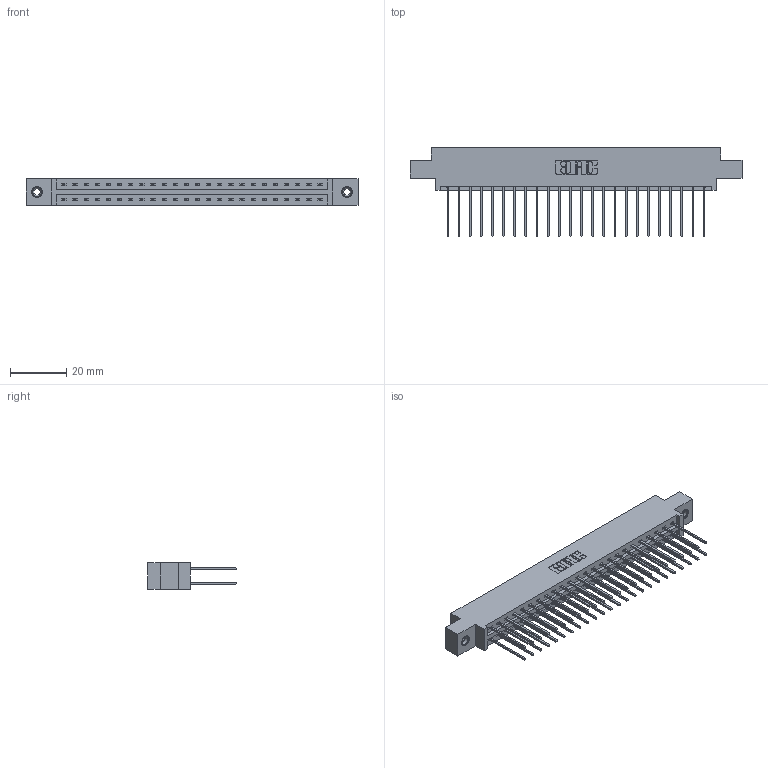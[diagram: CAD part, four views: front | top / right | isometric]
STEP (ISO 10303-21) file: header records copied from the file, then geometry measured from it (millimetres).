
FILE_DESCRIPTION (( 'STEP AP203' ), '1' );
FILE_NAME ('387-048-542-808.STEP', '2019-10-18T10:04:23', ( '' ), ( '' ), 'SwSTEP 2.0', 'SolidWorks 2016', '' );
FILE_SCHEMA (( 'CONFIG_CONTROL_DESIGN' ));
Length unit declared in the file: inch
Products named in the file (4): 345-292-001_345-293-142; 387-048-542-808; 337 Part_0.170 Offset - 0.156 Dia-TI; 345-250-001_345-250-003-102
Assembly tree (51 placements, depth 2):
  387-048-542-808
    337 Part_0.170 Offset - 0.156 Dia-TI
    345-292-001_345-293-142  x48
    345-250-001_345-250-003-102  x2
Bounding box: 118.11 x 31.63 x 9.4 mm (x, y, z)
Volume: 12307.5 mm3; surface area: 14986.1 mm2
Topology: 51 solids, 51 shells, 2770 faces, 8187 edges, 5386 vertices
Faces by surface type: plane 1930, cylinder 824, cone 12, torus 4
Entity records: 22272 total; most frequent: CARTESIAN_POINT 3749, ORIENTED_EDGE 3678, DIRECTION 3253, EDGE_CURVE 1839, VECTOR 1691, LINE 1691, VERTEX_POINT 1220, AXIS2_PLACEMENT_3D 781
